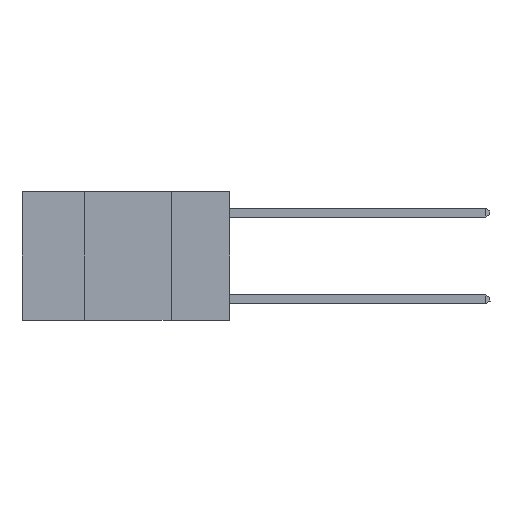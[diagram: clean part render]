
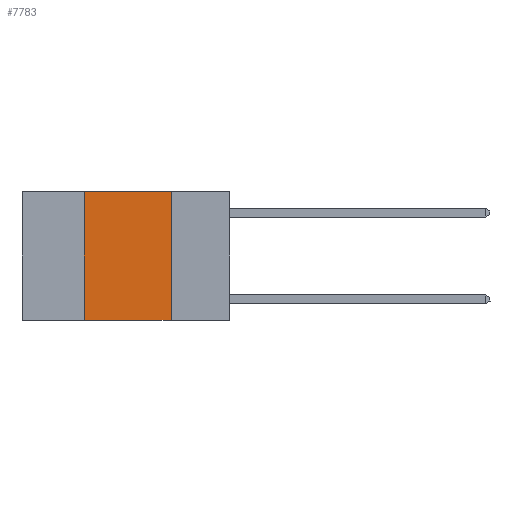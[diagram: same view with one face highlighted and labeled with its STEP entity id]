
A CAD part, left-side view. The second image highlights one B-rep face of the part: STEP entity #7783.
In plain terms, the highlighted planar face has unit normal (-1, 0, 0).
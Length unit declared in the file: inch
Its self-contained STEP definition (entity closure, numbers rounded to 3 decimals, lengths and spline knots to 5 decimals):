
#272 = ORIENTED_EDGE ( 'NONE', *, *, #11565, .F. ) ;
#333 = CARTESIAN_POINT ( 'NONE',  ( 0., 0.17, -0.37 ) ) ;
#339 = VECTOR ( 'NONE', #7223, 39.37008 ) ;
#383 = DIRECTION ( 'NONE',  ( 0., 0., -1. ) ) ;
#1107 = CARTESIAN_POINT ( 'NONE',  ( 0., 0.17, 0. ) ) ;
#1400 = LINE ( 'NONE', #18097, #13752 ) ;
#2563 = CARTESIAN_POINT ( 'NONE',  ( 0., 0.6, 0. ) ) ;
#2692 = DIRECTION ( 'NONE',  ( 0., 0., -1. ) ) ;
#3673 = DIRECTION ( 'NONE',  ( 0., -1., 0. ) ) ;
#5014 = PLANE ( 'NONE',  #12720 ) ;
#5565 = VERTEX_POINT ( 'NONE', #333 ) ;
#5834 = VECTOR ( 'NONE', #3673, 39.37008 ) ;
#5865 = LINE ( 'NONE', #14214, #5834 ) ;
#6305 = VECTOR ( 'NONE', #2692, 39.37008 ) ;
#7223 = DIRECTION ( 'NONE',  ( 0., 0., 1. ) ) ;
#7783 = ADVANCED_FACE ( 'NONE', ( #13103 ), #5014, .F. ) ;
#8987 = CARTESIAN_POINT ( 'NONE',  ( 0., 0.17, 0. ) ) ;
#10853 = EDGE_CURVE ( 'NONE', #24353, #18340, #5865, .T. ) ;
#11565 = EDGE_CURVE ( 'NONE', #18340, #5565, #21409, .T. ) ;
#12720 = AXIS2_PLACEMENT_3D ( 'NONE', #2563, #15283, #383 ) ;
#13103 = FACE_OUTER_BOUND ( 'NONE', #20481, .T. ) ;
#13752 = VECTOR ( 'NONE', #16031, 39.37008 ) ;
#14214 = CARTESIAN_POINT ( 'NONE',  ( 0., 0.6, 0. ) ) ;
#14462 = CARTESIAN_POINT ( 'NONE',  ( 0., 0.42, 0. ) ) ;
#14761 = ORIENTED_EDGE ( 'NONE', *, *, #10853, .F. ) ;
#15283 = DIRECTION ( 'NONE',  ( 1., 0., 0. ) ) ;
#16031 = DIRECTION ( 'NONE',  ( 0., -1., 0. ) ) ;
#16728 = EDGE_CURVE ( 'NONE', #25641, #5565, #1400, .T. ) ;
#16783 = CARTESIAN_POINT ( 'NONE',  ( 0., 0.42, -0.37 ) ) ;
#17207 = CARTESIAN_POINT ( 'NONE',  ( 0., 0.42, 0. ) ) ;
#18097 = CARTESIAN_POINT ( 'NONE',  ( 0., 0.6, -0.37 ) ) ;
#18340 = VERTEX_POINT ( 'NONE', #1107 ) ;
#20481 = EDGE_LOOP ( 'NONE', ( #272, #14761, #21582, #23227 ) ) ;
#21409 = LINE ( 'NONE', #8987, #6305 ) ;
#21582 = ORIENTED_EDGE ( 'NONE', *, *, #23736, .F. ) ;
#23227 = ORIENTED_EDGE ( 'NONE', *, *, #16728, .T. ) ;
#23736 = EDGE_CURVE ( 'NONE', #25641, #24353, #23904, .T. ) ;
#23904 = LINE ( 'NONE', #17207, #339 ) ;
#24353 = VERTEX_POINT ( 'NONE', #14462 ) ;
#25641 = VERTEX_POINT ( 'NONE', #16783 ) ;
